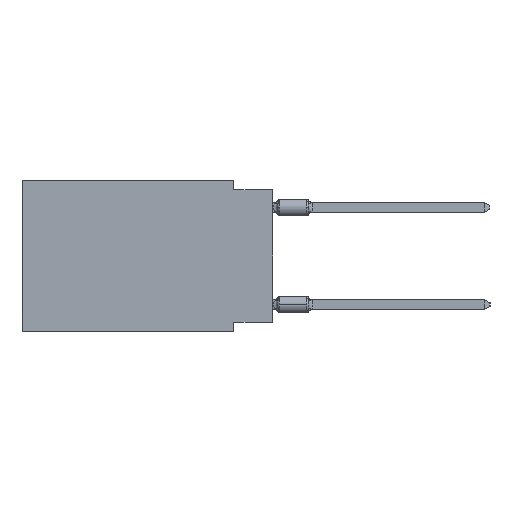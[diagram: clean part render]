
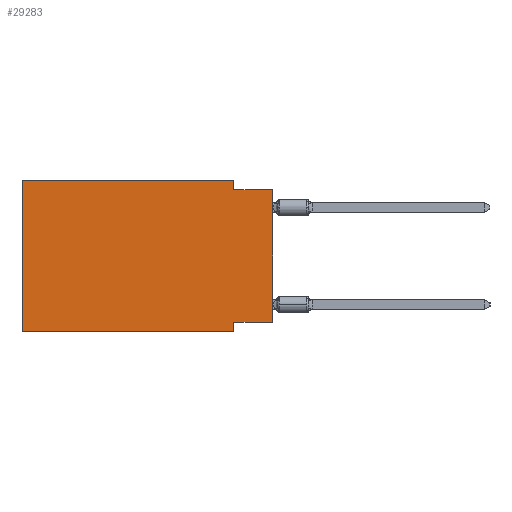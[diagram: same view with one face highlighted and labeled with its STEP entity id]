
A CAD part, left-side view. The second image highlights one B-rep face of the part: STEP entity #29283.
In plain terms, the highlighted planar face has unit normal (-1, 0, 0).
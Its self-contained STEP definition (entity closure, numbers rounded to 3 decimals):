
#482 = DIRECTION ( 'NONE',  ( 0., 0., -1. ) ) ;
#688 = VECTOR ( 'NONE', #25956, 1000. ) ;
#948 = EDGE_LOOP ( 'NONE', ( #3746, #30968, #34686, #20615, #13271, #36022, #23696, #34644 ) ) ;
#1157 = VERTEX_POINT ( 'NONE', #12777 ) ;
#2898 = CARTESIAN_POINT ( 'NONE',  ( 0., 2.54, 0. ) ) ;
#3746 = ORIENTED_EDGE ( 'NONE', *, *, #8666, .T. ) ;
#4078 = VECTOR ( 'NONE', #29588, 1000. ) ;
#4435 = VECTOR ( 'NONE', #22276, 1000. ) ;
#4820 = CARTESIAN_POINT ( 'NONE',  ( 0., 0., -9.271 ) ) ;
#5041 = CARTESIAN_POINT ( 'NONE',  ( 0., 16.383, -9.906 ) ) ;
#5324 = LINE ( 'NONE', #16666, #31294 ) ;
#6074 = LINE ( 'NONE', #36772, #15829 ) ;
#6291 = VECTOR ( 'NONE', #27719, 1000. ) ;
#6605 = LINE ( 'NONE', #28934, #688 ) ;
#6775 = CARTESIAN_POINT ( 'NONE',  ( 0., 16.383, 0. ) ) ;
#6929 = VERTEX_POINT ( 'NONE', #21149 ) ;
#8666 = EDGE_CURVE ( 'NONE', #9042, #29908, #28224, .T. ) ;
#9042 = VERTEX_POINT ( 'NONE', #25397 ) ;
#10370 = EDGE_CURVE ( 'NONE', #19982, #29908, #36655, .T. ) ;
#11176 = EDGE_CURVE ( 'NONE', #6929, #23887, #34812, .T. ) ;
#12163 = DIRECTION ( 'NONE',  ( 1., 0., 0. ) ) ;
#12777 = CARTESIAN_POINT ( 'NONE',  ( 0., 2.54, -9.271 ) ) ;
#13271 = ORIENTED_EDGE ( 'NONE', *, *, #24062, .F. ) ;
#13597 = CARTESIAN_POINT ( 'NONE',  ( 0., 2.54, -9.906 ) ) ;
#14062 = DIRECTION ( 'NONE',  ( 0., 0., 1. ) ) ;
#14588 = EDGE_CURVE ( 'NONE', #35281, #18321, #5324, .T. ) ;
#15829 = VECTOR ( 'NONE', #14062, 1000. ) ;
#16340 = LINE ( 'NONE', #4820, #29427 ) ;
#16666 = CARTESIAN_POINT ( 'NONE',  ( 0., 16.383, -9.906 ) ) ;
#17030 = VECTOR ( 'NONE', #482, 1000. ) ;
#17428 = CARTESIAN_POINT ( 'NONE',  ( 0., 2.54, -0.635 ) ) ;
#18321 = VERTEX_POINT ( 'NONE', #13597 ) ;
#18514 = AXIS2_PLACEMENT_3D ( 'NONE', #6775, #12163, #23532 ) ;
#18603 = CARTESIAN_POINT ( 'NONE',  ( 0., 2.54, 0. ) ) ;
#19177 = CARTESIAN_POINT ( 'NONE',  ( 0., 0., -0.635 ) ) ;
#19982 = VERTEX_POINT ( 'NONE', #17428 ) ;
#20615 = ORIENTED_EDGE ( 'NONE', *, *, #11176, .F. ) ;
#21149 = CARTESIAN_POINT ( 'NONE',  ( 0., 16.383, 0. ) ) ;
#22232 = EDGE_CURVE ( 'NONE', #9042, #1157, #16340, .T. ) ;
#22276 = DIRECTION ( 'NONE',  ( 0., 0., 1. ) ) ;
#23532 = DIRECTION ( 'NONE',  ( 0., 0., -1. ) ) ;
#23696 = ORIENTED_EDGE ( 'NONE', *, *, #29200, .F. ) ;
#23717 = PLANE ( 'NONE',  #18514 ) ;
#23887 = VERTEX_POINT ( 'NONE', #18603 ) ;
#24020 = EDGE_CURVE ( 'NONE', #23887, #19982, #33800, .T. ) ;
#24062 = EDGE_CURVE ( 'NONE', #35281, #6929, #6074, .T. ) ;
#25397 = CARTESIAN_POINT ( 'NONE',  ( 0., 0., -9.271 ) ) ;
#25956 = DIRECTION ( 'NONE',  ( 0., 0., -1. ) ) ;
#26319 = FACE_OUTER_BOUND ( 'NONE', #948, .T. ) ;
#27134 = DIRECTION ( 'NONE',  ( 0., 1., 0. ) ) ;
#27148 = CARTESIAN_POINT ( 'NONE',  ( 0., 16.383, 0. ) ) ;
#27719 = DIRECTION ( 'NONE',  ( 0., -1., 0. ) ) ;
#27860 = CARTESIAN_POINT ( 'NONE',  ( 0., 0., 0. ) ) ;
#28018 = DIRECTION ( 'NONE',  ( 0., -1., 0. ) ) ;
#28224 = LINE ( 'NONE', #27860, #4435 ) ;
#28934 = CARTESIAN_POINT ( 'NONE',  ( 0., 2.54, -9.906 ) ) ;
#29200 = EDGE_CURVE ( 'NONE', #1157, #18321, #6605, .T. ) ;
#29283 = ADVANCED_FACE ( 'NONE', ( #26319 ), #23717, .F. ) ;
#29427 = VECTOR ( 'NONE', #27134, 1000. ) ;
#29588 = DIRECTION ( 'NONE',  ( 0., -1., 0. ) ) ;
#29908 = VERTEX_POINT ( 'NONE', #19177 ) ;
#30968 = ORIENTED_EDGE ( 'NONE', *, *, #10370, .F. ) ;
#31294 = VECTOR ( 'NONE', #28018, 1000. ) ;
#33800 = LINE ( 'NONE', #2898, #17030 ) ;
#34644 = ORIENTED_EDGE ( 'NONE', *, *, #22232, .F. ) ;
#34686 = ORIENTED_EDGE ( 'NONE', *, *, #24020, .F. ) ;
#34812 = LINE ( 'NONE', #27148, #4078 ) ;
#35281 = VERTEX_POINT ( 'NONE', #5041 ) ;
#36022 = ORIENTED_EDGE ( 'NONE', *, *, #14588, .T. ) ;
#36286 = CARTESIAN_POINT ( 'NONE',  ( 0., 0., -0.635 ) ) ;
#36655 = LINE ( 'NONE', #36286, #6291 ) ;
#36772 = CARTESIAN_POINT ( 'NONE',  ( 0., 16.383, 0. ) ) ;
